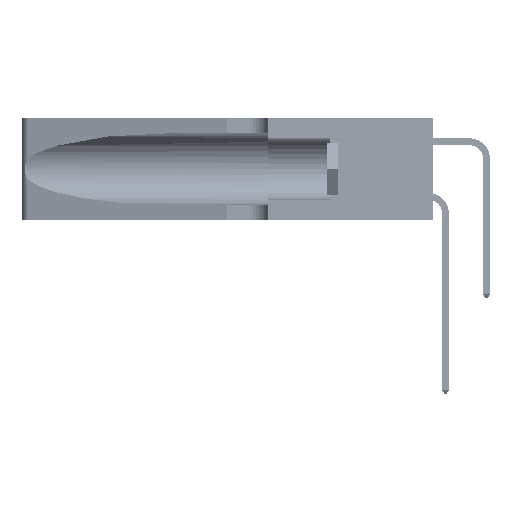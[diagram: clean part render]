
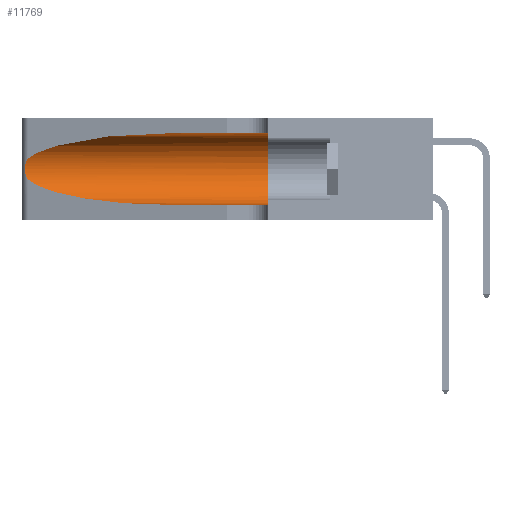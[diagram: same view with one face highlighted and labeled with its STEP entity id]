
A CAD part, left-side view. The second image highlights one B-rep face of the part: STEP entity #11769.
In plain terms, the highlighted cylindrical face has radius 3.308 mm (diameter 6.617 mm), a partial arc.
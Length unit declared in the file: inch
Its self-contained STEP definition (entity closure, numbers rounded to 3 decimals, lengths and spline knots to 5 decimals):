
#1346 = FACE_OUTER_BOUND ( 'NONE', #19102, .T. ) ;
#2574 = EDGE_CURVE ( 'NONE', #34479, #25514, #49838, .T. ) ;
#3246 = CARTESIAN_POINT ( 'NONE',  ( 0.1305, 1.61858, 0.05475 ) ) ;
#3500 = EDGE_CURVE ( 'NONE', #30382, #52094, #40556, .T. ) ;
#3505 = CARTESIAN_POINT ( 'NONE',  ( 0.1305, 0.35, 0.185 ) ) ;
#3589 = CARTESIAN_POINT ( 'NONE',  ( 0.26017, 1.23833, 0.17102 ) ) ;
#3885 = CARTESIAN_POINT ( 'NONE',  ( 0.1305, 0.72297, 0.31525 ) ) ;
#5100 = ORIENTED_EDGE ( 'NONE', *, *, #43668, .T. ) ;
#5732 = AXIS2_PLACEMENT_3D ( 'NONE', #38278, #12654, #21343 ) ;
#7825 = CARTESIAN_POINT ( 'NONE',  ( 0.1305, 0.72297, 0.05475 ) ) ;
#7828 = CARTESIAN_POINT ( 'NONE',  ( 0.25639, 1.23184, 0.21858 ) ) ;
#7936 = DIRECTION ( 'NONE',  ( 0., 0., 1. ) ) ;
#8019 = CARTESIAN_POINT ( 'NONE',  ( 0.25789, 1.23486, 0.15765 ) ) ;
#11769 = ADVANCED_FACE ( 'NONE', ( #1346 ), #25069, .F. ) ;
#12176 = CARTESIAN_POINT ( 'NONE',  ( 0.18966, 0.96281, 0.05475 ) ) ;
#12263 = CARTESIAN_POINT ( 'NONE',  ( 0.25555, 1.22994, 0.2215 ) ) ;
#12434 = CARTESIAN_POINT ( 'NONE',  ( 0.1305, 1.61858, 0.31525 ) ) ;
#12447 = CARTESIAN_POINT ( 'NONE',  ( 0.25555, 1.22993, 0.14849 ) ) ;
#12654 = DIRECTION ( 'NONE',  ( 0., -1., 0. ) ) ;
#12746 = CARTESIAN_POINT ( 'NONE',  ( 0.25487, 1.22718, 0.22369 ) ) ;
#16547 = ORIENTED_EDGE ( 'NONE', *, *, #18635, .T. ) ;
#18635 = EDGE_CURVE ( 'NONE', #50095, #30382, #38146, .T. ) ;
#19102 = EDGE_LOOP ( 'NONE', ( #16547, #39566, #5100, #47613, #38293, #44841 ) ) ;
#20957 = CARTESIAN_POINT ( 'NONE',  ( 0.25787, 1.23484, 0.2124 ) ) ;
#21322 = VECTOR ( 'NONE', #38065, 39.37008 ) ;
#21343 = DIRECTION ( 'NONE',  ( 0., 0., -1. ) ) ;
#25069 = CYLINDRICAL_SURFACE ( 'NONE', #5732, 0.13025 ) ;
#25236 = CARTESIAN_POINT ( 'NONE',  ( 0.26018, 1.23835, 0.19895 ) ) ;
#25514 = VERTEX_POINT ( 'NONE', #53607 ) ;
#29407 = CARTESIAN_POINT ( 'NONE',  ( 0.1305, 0.72297, 0.31525 ) ) ;
#29512 = CARTESIAN_POINT ( 'NONE',  ( 0.26075, 1.23896, 0.178 ) ) ;
#29566 = EDGE_CURVE ( 'NONE', #35965, #25514, #30818, .T. ) ;
#29795 = CARTESIAN_POINT ( 'NONE',  ( 0.18966, 0.96281, 0.31525 ) ) ;
#30382 = VERTEX_POINT ( 'NONE', #51051 ) ;
#30818 = LINE ( 'NONE', #3246, #44793 ) ;
#33480 = DIRECTION ( 'NONE',  ( 0., -1., 0. ) ) ;
#33540 = CARTESIAN_POINT ( 'NONE',  ( 0.25487, 1.22718, 0.14631 ) ) ;
#33732 = DIRECTION ( 'NONE',  ( 0., 1., 0. ) ) ;
#33807 = CARTESIAN_POINT ( 'NONE',  ( 0.25856, 1.23593, 0.16098 ) ) ;
#33890 = CARTESIAN_POINT ( 'NONE',  ( 0.25487, 1.22718, 0.14631 ) ) ;
#34479 = VERTEX_POINT ( 'NONE', #36724 ) ;
#35965 = VERTEX_POINT ( 'NONE', #7825 ) ;
#36724 = CARTESIAN_POINT ( 'NONE',  ( 0.1305, 0.35, 0.31525 ) ) ;
#37805 = CARTESIAN_POINT ( 'NONE',  ( 0.2373, 1.15595, 0.08982 ) ) ;
#38065 = DIRECTION ( 'NONE',  ( 0., -1., 0. ) ) ;
#38073 = CARTESIAN_POINT ( 'NONE',  ( 0.25639, 1.23186, 0.15144 ) ) ;
#38146 =( BOUNDED_CURVE ( )  B_SPLINE_CURVE ( 3, ( #3885, #29795, #38365, #12746 ),
 .UNSPECIFIED., .F., .T. ) 
 B_SPLINE_CURVE_WITH_KNOTS ( ( 4, 4 ),
 ( 1.5708, 2.84003 ),
 .UNSPECIFIED. ) 
 CURVE ( )  GEOMETRIC_REPRESENTATION_ITEM ( )  RATIONAL_B_SPLINE_CURVE ( ( 1., 0.87, 0.87, 1. ) ) 
 REPRESENTATION_ITEM ( '' )  );
#38278 = CARTESIAN_POINT ( 'NONE',  ( 0.1305, 1.61858, 0.185 ) ) ;
#38293 = ORIENTED_EDGE ( 'NONE', *, *, #2574, .F. ) ;
#38365 = CARTESIAN_POINT ( 'NONE',  ( 0.2373, 1.15595, 0.28018 ) ) ;
#39566 = ORIENTED_EDGE ( 'NONE', *, *, #3500, .T. ) ;
#39666 = EDGE_CURVE ( 'NONE', #50095, #34479, #45287, .T. ) ;
#40556 = B_SPLINE_CURVE_WITH_KNOTS ( 'NONE', 3,
 ( #46444, #12263, #7828, #20957, #50713, #25236, #54988, #29512, #3589, #33807, #8019, #38073, #12447, #42358 ),
 .UNSPECIFIED., .F., .F.,
 ( 4, 2, 2, 2, 2, 2, 4 ),
 ( 0., 0.00027, 0.00053, 0.00107, 0.0016, 0.00187, 0.00214 ),
 .UNSPECIFIED. ) ;
#41075 = AXIS2_PLACEMENT_3D ( 'NONE', #3505, #33732, #7936 ) ;
#42091 = CARTESIAN_POINT ( 'NONE',  ( 0.1305, 0.72297, 0.05475 ) ) ;
#42358 = CARTESIAN_POINT ( 'NONE',  ( 0.25487, 1.22718, 0.14631 ) ) ;
#43668 = EDGE_CURVE ( 'NONE', #52094, #35965, #48051, .T. ) ;
#44793 = VECTOR ( 'NONE', #33480, 39.37008 ) ;
#44841 = ORIENTED_EDGE ( 'NONE', *, *, #39666, .F. ) ;
#45287 = LINE ( 'NONE', #12434, #21322 ) ;
#46444 = CARTESIAN_POINT ( 'NONE',  ( 0.25487, 1.22718, 0.22369 ) ) ;
#47613 = ORIENTED_EDGE ( 'NONE', *, *, #29566, .T. ) ;
#48051 =( BOUNDED_CURVE ( )  B_SPLINE_CURVE ( 3, ( #33540, #37805, #12176, #42091 ),
 .UNSPECIFIED., .F., .F. ) 
 B_SPLINE_CURVE_WITH_KNOTS ( ( 4, 4 ),
 ( 3.44316, 4.71239 ),
 .UNSPECIFIED. ) 
 CURVE ( )  GEOMETRIC_REPRESENTATION_ITEM ( )  RATIONAL_B_SPLINE_CURVE ( ( 1., 0.87, 0.87, 1. ) ) 
 REPRESENTATION_ITEM ( '' )  );
#49838 = CIRCLE ( 'NONE', #41075, 0.13025 ) ;
#50095 = VERTEX_POINT ( 'NONE', #29407 ) ;
#50713 = CARTESIAN_POINT ( 'NONE',  ( 0.25854, 1.2359, 0.20912 ) ) ;
#51051 = CARTESIAN_POINT ( 'NONE',  ( 0.25487, 1.22718, 0.22369 ) ) ;
#52094 = VERTEX_POINT ( 'NONE', #33890 ) ;
#53607 = CARTESIAN_POINT ( 'NONE',  ( 0.1305, 0.35, 0.05475 ) ) ;
#54988 = CARTESIAN_POINT ( 'NONE',  ( 0.26075, 1.23896, 0.19203 ) ) ;
